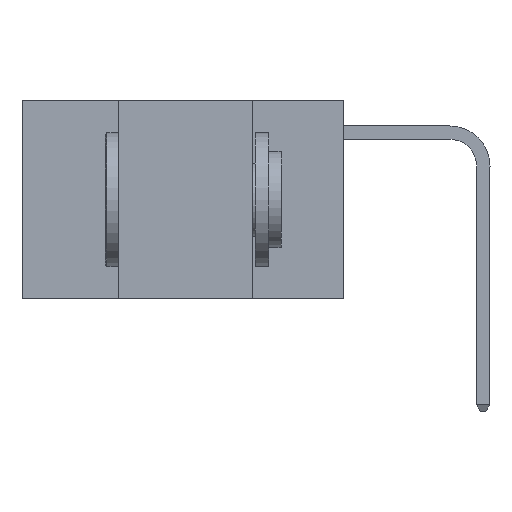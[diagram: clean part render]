
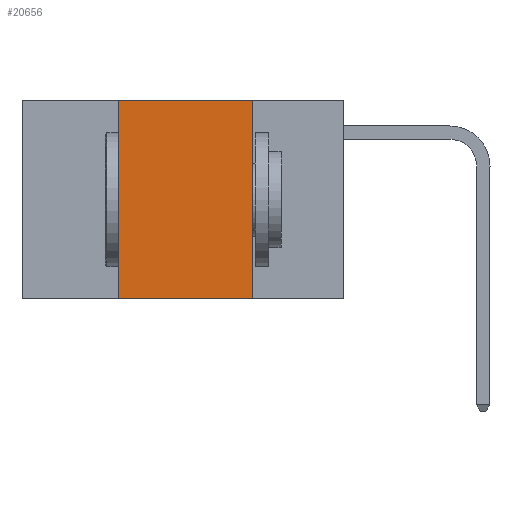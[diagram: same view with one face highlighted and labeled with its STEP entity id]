
A CAD part, left-side view. The second image highlights one B-rep face of the part: STEP entity #20656.
In plain terms, the highlighted planar face has unit normal (-1, 0, 0).
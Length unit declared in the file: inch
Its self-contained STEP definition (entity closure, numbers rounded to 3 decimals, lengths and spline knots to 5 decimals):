
#30 = LINE ( 'NONE', #9940, #2085 ) ;
#338 = FACE_OUTER_BOUND ( 'NONE', #9118, .T. ) ;
#411 = EDGE_CURVE ( 'NONE', #17644, #5716, #17175, .T. ) ;
#1473 = ORIENTED_EDGE ( 'NONE', *, *, #411, .F. ) ;
#1734 = DIRECTION ( 'NONE',  ( 0., -1., 0. ) ) ;
#2085 = VECTOR ( 'NONE', #1734, 39.37008 ) ;
#2399 = CARTESIAN_POINT ( 'NONE',  ( 0., 0.6, 0. ) ) ;
#2601 = CARTESIAN_POINT ( 'NONE',  ( 0., 0.42, 0. ) ) ;
#4021 = DIRECTION ( 'NONE',  ( 0., 0., -1. ) ) ;
#4114 = VECTOR ( 'NONE', #8421, 39.37008 ) ;
#4793 = ORIENTED_EDGE ( 'NONE', *, *, #9839, .F. ) ;
#5716 = VERTEX_POINT ( 'NONE', #2601 ) ;
#6146 = DIRECTION ( 'NONE',  ( 0., 0., -1. ) ) ;
#6905 = CARTESIAN_POINT ( 'NONE',  ( 0., 0.17, -0.37 ) ) ;
#7199 = PLANE ( 'NONE',  #13492 ) ;
#7370 = ORIENTED_EDGE ( 'NONE', *, *, #11660, .F. ) ;
#8421 = DIRECTION ( 'NONE',  ( 0., 0., 1. ) ) ;
#8523 = CARTESIAN_POINT ( 'NONE',  ( 0., 0.42, 0. ) ) ;
#9118 = EDGE_LOOP ( 'NONE', ( #7370, #4793, #1473, #16599 ) ) ;
#9839 = EDGE_CURVE ( 'NONE', #5716, #10115, #11374, .T. ) ;
#9940 = CARTESIAN_POINT ( 'NONE',  ( 0., 0.6, -0.37 ) ) ;
#10115 = VERTEX_POINT ( 'NONE', #11783 ) ;
#10299 = VECTOR ( 'NONE', #6146, 39.37008 ) ;
#11207 = CARTESIAN_POINT ( 'NONE',  ( 0., 0.42, -0.37 ) ) ;
#11374 = LINE ( 'NONE', #14312, #19490 ) ;
#11660 = EDGE_CURVE ( 'NONE', #10115, #17527, #14623, .T. ) ;
#11783 = CARTESIAN_POINT ( 'NONE',  ( 0., 0.17, 0. ) ) ;
#13492 = AXIS2_PLACEMENT_3D ( 'NONE', #2399, #13847, #4021 ) ;
#13847 = DIRECTION ( 'NONE',  ( 1., 0., 0. ) ) ;
#13984 = EDGE_CURVE ( 'NONE', #17644, #17527, #30, .T. ) ;
#14312 = CARTESIAN_POINT ( 'NONE',  ( 0., 0.6, 0. ) ) ;
#14623 = LINE ( 'NONE', #20733, #10299 ) ;
#15956 = DIRECTION ( 'NONE',  ( 0., -1., 0. ) ) ;
#16599 = ORIENTED_EDGE ( 'NONE', *, *, #13984, .T. ) ;
#17175 = LINE ( 'NONE', #8523, #4114 ) ;
#17527 = VERTEX_POINT ( 'NONE', #6905 ) ;
#17644 = VERTEX_POINT ( 'NONE', #11207 ) ;
#19490 = VECTOR ( 'NONE', #15956, 39.37008 ) ;
#20656 = ADVANCED_FACE ( 'NONE', ( #338 ), #7199, .F. ) ;
#20733 = CARTESIAN_POINT ( 'NONE',  ( 0., 0.17, 0. ) ) ;
